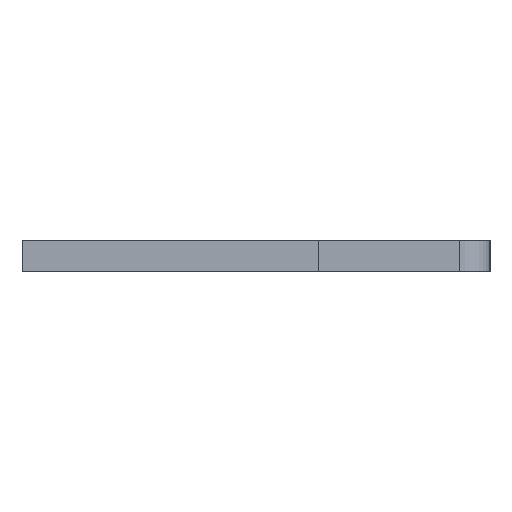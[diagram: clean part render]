
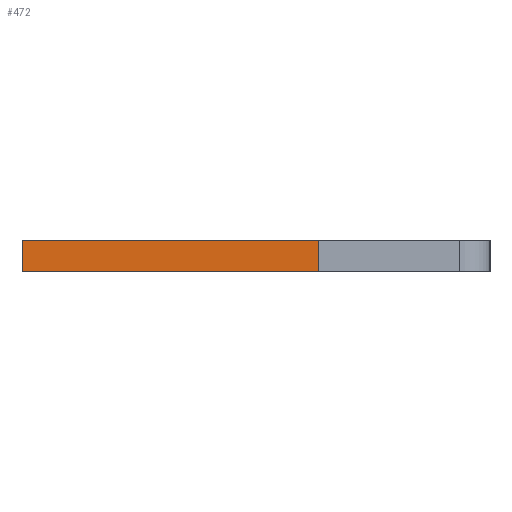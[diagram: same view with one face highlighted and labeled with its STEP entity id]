
A CAD part, left-side view. The second image highlights one B-rep face of the part: STEP entity #472.
In plain terms, the highlighted face is planar.
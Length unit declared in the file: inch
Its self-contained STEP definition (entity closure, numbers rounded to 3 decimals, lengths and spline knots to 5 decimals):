
#80 = VECTOR ( 'NONE', #1053, 39.37008 ) ;
#93 = LINE ( 'NONE', #1431, #874 ) ;
#100 = CARTESIAN_POINT ( 'NONE',  ( -0.01, 0.15, -0.04 ) ) ;
#134 = VERTEX_POINT ( 'NONE', #1153 ) ;
#163 = EDGE_CURVE ( 'NONE', #134, #309, #93, .T. ) ;
#210 = ORIENTED_EDGE ( 'NONE', *, *, #330, .F. ) ;
#212 = DIRECTION ( 'NONE',  ( -1., 0., 0. ) ) ;
#309 = VERTEX_POINT ( 'NONE', #100 ) ;
#322 = ORIENTED_EDGE ( 'NONE', *, *, #1550, .T. ) ;
#330 = EDGE_CURVE ( 'NONE', #1136, #134, #463, .T. ) ;
#352 = VERTEX_POINT ( 'NONE', #633 ) ;
#385 = PLANE ( 'NONE',  #945 ) ;
#463 = LINE ( 'NONE', #1328, #80 ) ;
#472 = ADVANCED_FACE ( 'NONE', ( #1510 ), #385, .F. ) ;
#473 = CARTESIAN_POINT ( 'NONE',  ( -0.01, 0.15, -0.04 ) ) ;
#550 = VECTOR ( 'NONE', #999, 39.37008 ) ;
#633 = CARTESIAN_POINT ( 'NONE',  ( -0.01, -0.04, -0.04 ) ) ;
#641 = DIRECTION ( 'NONE',  ( 0., 0., 1. ) ) ;
#703 = CARTESIAN_POINT ( 'NONE',  ( 0.01, -0.04, -0.04 ) ) ;
#850 = VECTOR ( 'NONE', #212, 39.37008 ) ;
#874 = VECTOR ( 'NONE', #1681, 39.37008 ) ;
#945 = AXIS2_PLACEMENT_3D ( 'NONE', #1451, #641, #1568 ) ;
#992 = CARTESIAN_POINT ( 'NONE',  ( 0.01, -0.04, -0.04 ) ) ;
#999 = DIRECTION ( 'NONE',  ( 0., 1., 0. ) ) ;
#1053 = DIRECTION ( 'NONE',  ( 0., 1., 0. ) ) ;
#1120 = ORIENTED_EDGE ( 'NONE', *, *, #1406, .T. ) ;
#1136 = VERTEX_POINT ( 'NONE', #703 ) ;
#1153 = CARTESIAN_POINT ( 'NONE',  ( 0.01, 0.15, -0.04 ) ) ;
#1228 = ORIENTED_EDGE ( 'NONE', *, *, #163, .F. ) ;
#1267 = LINE ( 'NONE', #992, #850 ) ;
#1328 = CARTESIAN_POINT ( 'NONE',  ( 0.01, 0.15, -0.04 ) ) ;
#1353 = LINE ( 'NONE', #473, #550 ) ;
#1406 = EDGE_CURVE ( 'NONE', #352, #309, #1353, .T. ) ;
#1419 = EDGE_LOOP ( 'NONE', ( #1120, #1228, #210, #322 ) ) ;
#1431 = CARTESIAN_POINT ( 'NONE',  ( 0.01, 0.15, -0.04 ) ) ;
#1451 = CARTESIAN_POINT ( 'NONE',  ( 0.01, 0.15, -0.04 ) ) ;
#1510 = FACE_OUTER_BOUND ( 'NONE', #1419, .T. ) ;
#1550 = EDGE_CURVE ( 'NONE', #1136, #352, #1267, .T. ) ;
#1568 = DIRECTION ( 'NONE',  ( 1., 0., 0. ) ) ;
#1681 = DIRECTION ( 'NONE',  ( -1., 0., 0. ) ) ;
